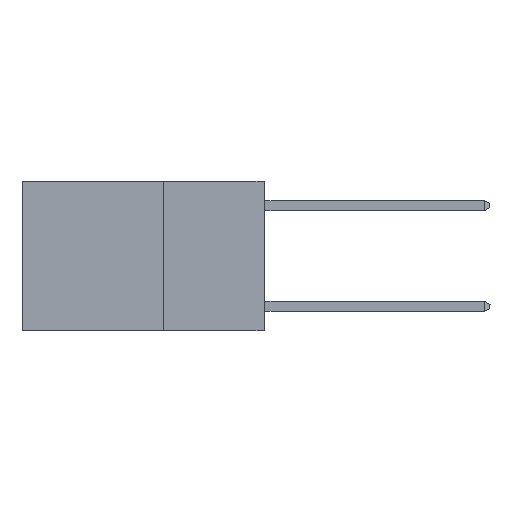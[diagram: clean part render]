
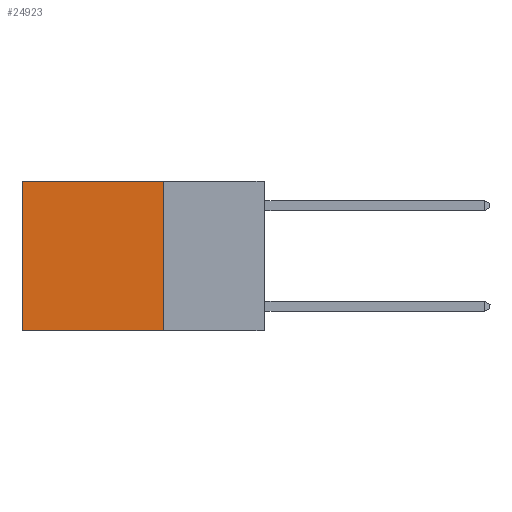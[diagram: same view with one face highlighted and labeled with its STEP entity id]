
A CAD part, left-side view. The second image highlights one B-rep face of the part: STEP entity #24923.
In plain terms, the highlighted planar face has unit normal (-1, 0, 0).
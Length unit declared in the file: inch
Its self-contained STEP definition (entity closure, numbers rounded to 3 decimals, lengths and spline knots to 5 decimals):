
#233 = CARTESIAN_POINT ( 'NONE',  ( 0.2625, 0.6, 0. ) ) ;
#2830 = DIRECTION ( 'NONE',  ( 0., 1., 0. ) ) ;
#3169 = DIRECTION ( 'NONE',  ( 0., 0., -1. ) ) ;
#3500 = LINE ( 'NONE', #8926, #27824 ) ;
#3676 = DIRECTION ( 'NONE',  ( 0., 0., -1. ) ) ;
#3688 = CARTESIAN_POINT ( 'NONE',  ( 0.2625, 0.25, -0.37 ) ) ;
#5583 = VERTEX_POINT ( 'NONE', #10680 ) ;
#5854 = LINE ( 'NONE', #28726, #11247 ) ;
#6153 = EDGE_CURVE ( 'NONE', #5583, #17772, #5854, .T. ) ;
#7462 = CARTESIAN_POINT ( 'NONE',  ( 0.2625, 0.6, -0.37 ) ) ;
#8926 = CARTESIAN_POINT ( 'NONE',  ( 0.2625, 0.25, 0. ) ) ;
#9173 = VECTOR ( 'NONE', #13994, 39.37008 ) ;
#10049 = PLANE ( 'NONE',  #21161 ) ;
#10680 = CARTESIAN_POINT ( 'NONE',  ( 0.2625, 0.25, 0. ) ) ;
#10848 = ORIENTED_EDGE ( 'NONE', *, *, #6153, .F. ) ;
#11247 = VECTOR ( 'NONE', #3676, 39.37008 ) ;
#13836 = EDGE_CURVE ( 'NONE', #17772, #19461, #28080, .T. ) ;
#13994 = DIRECTION ( 'NONE',  ( 0., 0., -1. ) ) ;
#15206 = LINE ( 'NONE', #233, #9173 ) ;
#16204 = CARTESIAN_POINT ( 'NONE',  ( 0.2625, 0.6, 0. ) ) ;
#16931 = DIRECTION ( 'NONE',  ( 1., 0., 0. ) ) ;
#16936 = ORIENTED_EDGE ( 'NONE', *, *, #18622, .T. ) ;
#17772 = VERTEX_POINT ( 'NONE', #3688 ) ;
#18622 = EDGE_CURVE ( 'NONE', #5583, #25394, #3500, .T. ) ;
#18795 = EDGE_CURVE ( 'NONE', #25394, #19461, #15206, .T. ) ;
#19160 = FACE_OUTER_BOUND ( 'NONE', #26601, .T. ) ;
#19461 = VERTEX_POINT ( 'NONE', #7462 ) ;
#21161 = AXIS2_PLACEMENT_3D ( 'NONE', #21409, #16931, #3169 ) ;
#21409 = CARTESIAN_POINT ( 'NONE',  ( 0.2625, 0.25, 0. ) ) ;
#22047 = VECTOR ( 'NONE', #2830, 39.37008 ) ;
#22829 = ORIENTED_EDGE ( 'NONE', *, *, #18795, .T. ) ;
#24886 = DIRECTION ( 'NONE',  ( 0., 1., 0. ) ) ;
#24911 = ORIENTED_EDGE ( 'NONE', *, *, #13836, .F. ) ;
#24923 = ADVANCED_FACE ( 'NONE', ( #19160 ), #10049, .F. ) ;
#25394 = VERTEX_POINT ( 'NONE', #16204 ) ;
#26601 = EDGE_LOOP ( 'NONE', ( #22829, #24911, #10848, #16936 ) ) ;
#27824 = VECTOR ( 'NONE', #24886, 39.37008 ) ;
#28005 = CARTESIAN_POINT ( 'NONE',  ( 0.2625, 0.25, -0.37 ) ) ;
#28080 = LINE ( 'NONE', #28005, #22047 ) ;
#28726 = CARTESIAN_POINT ( 'NONE',  ( 0.2625, 0.25, 0. ) ) ;
